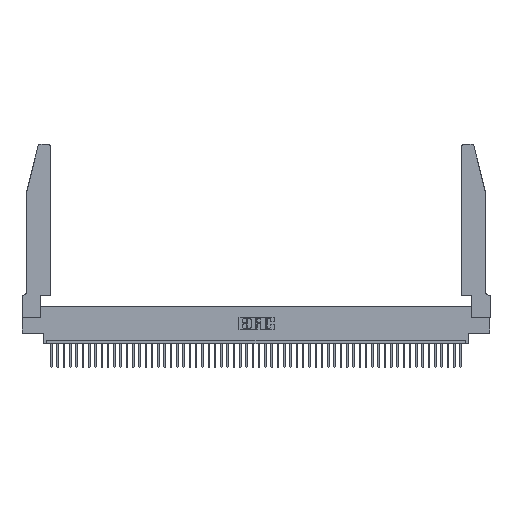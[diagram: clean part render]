
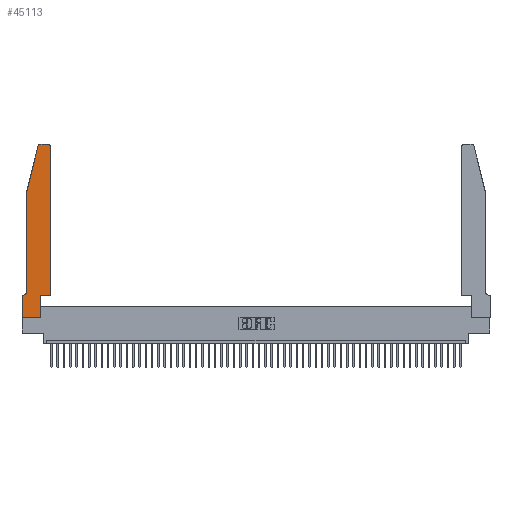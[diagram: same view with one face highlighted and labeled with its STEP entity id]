
A CAD part, top view. The second image highlights one B-rep face of the part: STEP entity #45113.
In plain terms, the highlighted planar face has unit normal (0, 0, 1).
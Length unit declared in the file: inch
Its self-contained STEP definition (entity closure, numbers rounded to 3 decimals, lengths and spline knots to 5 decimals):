
#295 = CARTESIAN_POINT ( 'NONE',  ( 0.0755, 0.42, 0.37 ) ) ;
#447 = DIRECTION ( 'NONE',  ( 1., 0., 0. ) ) ;
#1299 = LINE ( 'NONE', #20896, #46609 ) ;
#2314 = VERTEX_POINT ( 'NONE', #22579 ) ;
#2651 = CARTESIAN_POINT ( 'NONE',  ( 0.2865, 0.35, 0.37 ) ) ;
#3029 = ORIENTED_EDGE ( 'NONE', *, *, #44143, .T. ) ;
#3146 = FACE_OUTER_BOUND ( 'NONE', #21075, .T. ) ;
#4357 = VECTOR ( 'NONE', #13870, 39.37008 ) ;
#5640 = PLANE ( 'NONE',  #37294 ) ;
#5677 = DIRECTION ( 'NONE',  ( 0., 0., -1. ) ) ;
#6026 = VERTEX_POINT ( 'NONE', #15738 ) ;
#6174 = CARTESIAN_POINT ( 'NONE',  ( 0.0055, 0.42, 0.37 ) ) ;
#6273 = ORIENTED_EDGE ( 'NONE', *, *, #40525, .T. ) ;
#6962 = CARTESIAN_POINT ( 'NONE',  ( 0., 0.35, 0.37 ) ) ;
#7301 = EDGE_CURVE ( 'NONE', #49766, #30003, #34649, .T. ) ;
#8368 = VECTOR ( 'NONE', #8965, 39.37008 ) ;
#8965 = DIRECTION ( 'NONE',  ( 0., -1., 0. ) ) ;
#9520 = VERTEX_POINT ( 'NONE', #25364 ) ;
#9968 = DIRECTION ( 'NONE',  ( 0., 0., 1. ) ) ;
#10200 = AXIS2_PLACEMENT_3D ( 'NONE', #6174, #5677, #18060 ) ;
#10299 = ORIENTED_EDGE ( 'NONE', *, *, #12497, .T. ) ;
#11705 = CARTESIAN_POINT ( 'NONE',  ( 0.4505, 2.72, 0.37 ) ) ;
#12113 = CARTESIAN_POINT ( 'NONE',  ( 0.25487, 2.72718, 0.37 ) ) ;
#12254 = ORIENTED_EDGE ( 'NONE', *, *, #32426, .T. ) ;
#12497 = EDGE_CURVE ( 'NONE', #35842, #50907, #25157, .T. ) ;
#12628 = CARTESIAN_POINT ( 'NONE',  ( 0., 0., 0.37 ) ) ;
#12829 = CARTESIAN_POINT ( 'NONE',  ( 0.0755, 0.35, 0.37 ) ) ;
#12864 = CARTESIAN_POINT ( 'NONE',  ( 0., 0.35, 0.37 ) ) ;
#13222 = CARTESIAN_POINT ( 'NONE',  ( 0.284, 2.72, 0.37 ) ) ;
#13567 = DIRECTION ( 'NONE',  ( 1., 0., 0. ) ) ;
#13844 = CARTESIAN_POINT ( 'NONE',  ( 0., 0., 0.37 ) ) ;
#13870 = DIRECTION ( 'NONE',  ( -1., 0., 0. ) ) ;
#14633 = VECTOR ( 'NONE', #16565, 39.37008 ) ;
#14676 = EDGE_CURVE ( 'NONE', #9520, #48378, #17023, .T. ) ;
#14834 = LINE ( 'NONE', #12829, #4357 ) ;
#15092 = ORIENTED_EDGE ( 'NONE', *, *, #27703, .T. ) ;
#15738 = CARTESIAN_POINT ( 'NONE',  ( 0.4205, 2.75, 0.37 ) ) ;
#16565 = DIRECTION ( 'NONE',  ( 0., -1., 0. ) ) ;
#16804 = CARTESIAN_POINT ( 'NONE',  ( 0.0755, 2., 0.37 ) ) ;
#17023 = LINE ( 'NONE', #48199, #8368 ) ;
#18027 = CARTESIAN_POINT ( 'NONE',  ( 0.2865, 0.35, 0.37 ) ) ;
#18060 = DIRECTION ( 'NONE',  ( -1., 0., 0. ) ) ;
#18683 = AXIS2_PLACEMENT_3D ( 'NONE', #28288, #24110, #447 ) ;
#19274 = ORIENTED_EDGE ( 'NONE', *, *, #44389, .T. ) ;
#20046 = AXIS2_PLACEMENT_3D ( 'NONE', #13222, #9968, #13567 ) ;
#20896 = CARTESIAN_POINT ( 'NONE',  ( 0.2605, 2.75, 0.37 ) ) ;
#20997 = DIRECTION ( 'NONE',  ( 0., 0., 1. ) ) ;
#21075 = EDGE_LOOP ( 'NONE', ( #19274, #10299, #15092, #50990, #50320, #46513, #6273, #30394, #47826, #12254, #3029, #32187 ) ) ;
#21333 = VERTEX_POINT ( 'NONE', #6962 ) ;
#21738 = VECTOR ( 'NONE', #33974, 39.37008 ) ;
#22579 = CARTESIAN_POINT ( 'NONE',  ( 0.4505, 0.35, 0.37 ) ) ;
#22737 = LINE ( 'NONE', #22815, #40757 ) ;
#22769 = DIRECTION ( 'NONE',  ( -0.239, -0.971, 0. ) ) ;
#22815 = CARTESIAN_POINT ( 'NONE',  ( 0.4505, 0.35, 0.37 ) ) ;
#24110 = DIRECTION ( 'NONE',  ( 0., 0., 1. ) ) ;
#25157 = CIRCLE ( 'NONE', #20046, 0.03 ) ;
#25364 = CARTESIAN_POINT ( 'NONE',  ( 0.0755, 2., 0.37 ) ) ;
#26716 = CARTESIAN_POINT ( 'NONE',  ( 0., 0., 0.37 ) ) ;
#27703 = EDGE_CURVE ( 'NONE', #50907, #9520, #50559, .T. ) ;
#28288 = CARTESIAN_POINT ( 'NONE',  ( 0.4205, 2.72, 0.37 ) ) ;
#29194 = CIRCLE ( 'NONE', #10200, 0.07 ) ;
#30003 = VERTEX_POINT ( 'NONE', #2651 ) ;
#30394 = ORIENTED_EDGE ( 'NONE', *, *, #35951, .T. ) ;
#30642 = VERTEX_POINT ( 'NONE', #50123 ) ;
#30735 = VECTOR ( 'NONE', #33585, 39.37008 ) ;
#32110 = VERTEX_POINT ( 'NONE', #26716 ) ;
#32187 = ORIENTED_EDGE ( 'NONE', *, *, #34780, .T. ) ;
#32420 = VECTOR ( 'NONE', #22769, 39.37008 ) ;
#32426 = EDGE_CURVE ( 'NONE', #30003, #2314, #22737, .T. ) ;
#33585 = DIRECTION ( 'NONE',  ( 1., 0., 0. ) ) ;
#33631 = EDGE_CURVE ( 'NONE', #30642, #21333, #14834, .T. ) ;
#33974 = DIRECTION ( 'NONE',  ( 0., 1., 0. ) ) ;
#34649 = LINE ( 'NONE', #18027, #41489 ) ;
#34780 = EDGE_CURVE ( 'NONE', #43267, #6026, #46378, .T. ) ;
#35833 = CARTESIAN_POINT ( 'NONE',  ( 0.2865, 0., 0.37 ) ) ;
#35842 = VERTEX_POINT ( 'NONE', #36597 ) ;
#35951 = EDGE_CURVE ( 'NONE', #32110, #49766, #45599, .T. ) ;
#36378 = DIRECTION ( 'NONE',  ( -1., 0., 0. ) ) ;
#36597 = CARTESIAN_POINT ( 'NONE',  ( 0.284, 2.75, 0.37 ) ) ;
#36673 = DIRECTION ( 'NONE',  ( 1., 0., 0. ) ) ;
#37294 = AXIS2_PLACEMENT_3D ( 'NONE', #12864, #20997, #36673 ) ;
#38035 = DIRECTION ( 'NONE',  ( 0., 1., 0. ) ) ;
#38549 = CARTESIAN_POINT ( 'NONE',  ( 0.4505, 0.35, 0.37 ) ) ;
#39186 = LINE ( 'NONE', #38549, #21738 ) ;
#40525 = EDGE_CURVE ( 'NONE', #21333, #32110, #48806, .T. ) ;
#40757 = VECTOR ( 'NONE', #46419, 39.37008 ) ;
#41489 = VECTOR ( 'NONE', #38035, 39.37008 ) ;
#43267 = VERTEX_POINT ( 'NONE', #11705 ) ;
#44143 = EDGE_CURVE ( 'NONE', #2314, #43267, #39186, .T. ) ;
#44389 = EDGE_CURVE ( 'NONE', #6026, #35842, #1299, .T. ) ;
#45113 = ADVANCED_FACE ( 'NONE', ( #3146 ), #5640, .T. ) ;
#45599 = LINE ( 'NONE', #13844, #30735 ) ;
#46378 = CIRCLE ( 'NONE', #18683, 0.03 ) ;
#46419 = DIRECTION ( 'NONE',  ( 1., 0., 0. ) ) ;
#46513 = ORIENTED_EDGE ( 'NONE', *, *, #33631, .T. ) ;
#46609 = VECTOR ( 'NONE', #36378, 39.37008 ) ;
#47826 = ORIENTED_EDGE ( 'NONE', *, *, #7301, .T. ) ;
#48199 = CARTESIAN_POINT ( 'NONE',  ( 0.0755, 2., 0.37 ) ) ;
#48378 = VERTEX_POINT ( 'NONE', #295 ) ;
#48806 = LINE ( 'NONE', #12628, #14633 ) ;
#49766 = VERTEX_POINT ( 'NONE', #35833 ) ;
#50029 = EDGE_CURVE ( 'NONE', #48378, #30642, #29194, .T. ) ;
#50123 = CARTESIAN_POINT ( 'NONE',  ( 0.0055, 0.35, 0.37 ) ) ;
#50320 = ORIENTED_EDGE ( 'NONE', *, *, #50029, .T. ) ;
#50559 = LINE ( 'NONE', #16804, #32420 ) ;
#50907 = VERTEX_POINT ( 'NONE', #12113 ) ;
#50990 = ORIENTED_EDGE ( 'NONE', *, *, #14676, .T. ) ;
